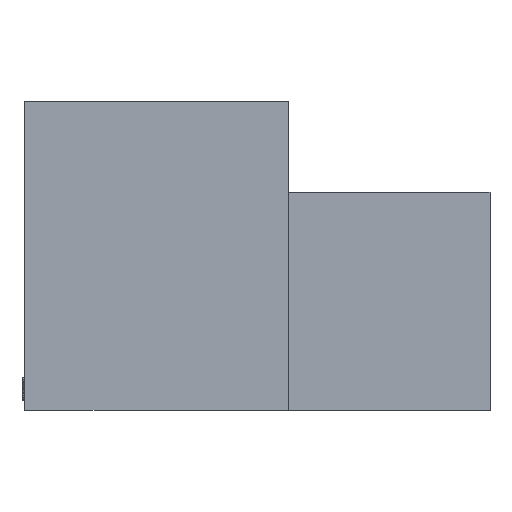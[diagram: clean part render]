
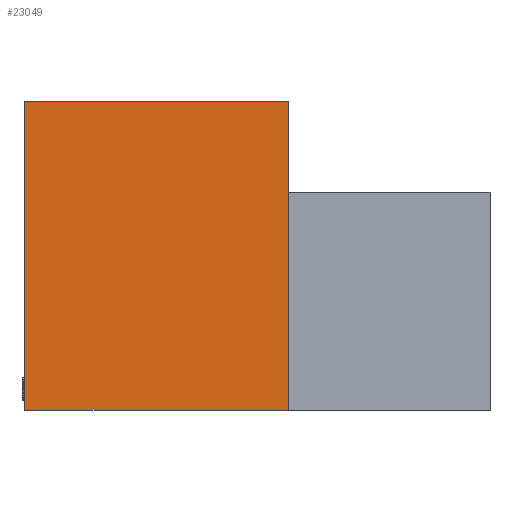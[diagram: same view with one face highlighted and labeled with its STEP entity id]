
A CAD part, left-side view. The second image highlights one B-rep face of the part: STEP entity #23049.
In plain terms, the highlighted planar face has unit normal (-1, 0, 0).
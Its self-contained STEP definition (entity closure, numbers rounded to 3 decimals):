
#2548 = ORIENTED_EDGE ( 'NONE', *, *, #28507, .F. ) ;
#4010 = EDGE_CURVE ( 'NONE', #14065, #12127, #7522, .T. ) ;
#5676 = VECTOR ( 'NONE', #15076, 1000. ) ;
#6004 = CARTESIAN_POINT ( 'NONE',  ( 0., 0., -13.487 ) ) ;
#7060 = CARTESIAN_POINT ( 'NONE',  ( 0., 0., 0. ) ) ;
#7522 = LINE ( 'NONE', #29493, #5676 ) ;
#7609 = CARTESIAN_POINT ( 'NONE',  ( 0., 11.506, 0. ) ) ;
#7716 = LINE ( 'NONE', #26022, #24656 ) ;
#8737 = ORIENTED_EDGE ( 'NONE', *, *, #4010, .F. ) ;
#9044 = EDGE_LOOP ( 'NONE', ( #2548, #8737, #27747, #22302 ) ) ;
#10040 = EDGE_CURVE ( 'NONE', #21466, #14065, #27737, .T. ) ;
#11107 = LINE ( 'NONE', #30777, #28053 ) ;
#12127 = VERTEX_POINT ( 'NONE', #6004 ) ;
#14065 = VERTEX_POINT ( 'NONE', #14375 ) ;
#14375 = CARTESIAN_POINT ( 'NONE',  ( 0., 0., 0. ) ) ;
#15076 = DIRECTION ( 'NONE',  ( 0., 0., -1. ) ) ;
#16360 = DIRECTION ( 'NONE',  ( 0., 1., 0. ) ) ;
#18876 = DIRECTION ( 'NONE',  ( 0., 0., 1. ) ) ;
#19859 = CARTESIAN_POINT ( 'NONE',  ( 0., 11.506, 0. ) ) ;
#21290 = AXIS2_PLACEMENT_3D ( 'NONE', #7060, #28750, #24002 ) ;
#21466 = VERTEX_POINT ( 'NONE', #7609 ) ;
#21581 = PLANE ( 'NONE',  #21290 ) ;
#22302 = ORIENTED_EDGE ( 'NONE', *, *, #28641, .F. ) ;
#22404 = DIRECTION ( 'NONE',  ( 0., -1., 0. ) ) ;
#23049 = ADVANCED_FACE ( 'NONE', ( #23378 ), #21581, .F. ) ;
#23378 = FACE_OUTER_BOUND ( 'NONE', #9044, .T. ) ;
#24002 = DIRECTION ( 'NONE',  ( 0., 0., -1. ) ) ;
#24093 = VERTEX_POINT ( 'NONE', #24475 ) ;
#24475 = CARTESIAN_POINT ( 'NONE',  ( 0., 11.506, -13.487 ) ) ;
#24656 = VECTOR ( 'NONE', #18876, 1000. ) ;
#26022 = CARTESIAN_POINT ( 'NONE',  ( 0., 11.506, -13.487 ) ) ;
#26199 = VECTOR ( 'NONE', #22404, 1000. ) ;
#27737 = LINE ( 'NONE', #19859, #26199 ) ;
#27747 = ORIENTED_EDGE ( 'NONE', *, *, #10040, .F. ) ;
#28053 = VECTOR ( 'NONE', #16360, 1000. ) ;
#28507 = EDGE_CURVE ( 'NONE', #12127, #24093, #11107, .T. ) ;
#28641 = EDGE_CURVE ( 'NONE', #24093, #21466, #7716, .T. ) ;
#28750 = DIRECTION ( 'NONE',  ( 1., 0., 0. ) ) ;
#29493 = CARTESIAN_POINT ( 'NONE',  ( 0., 0., 0. ) ) ;
#30777 = CARTESIAN_POINT ( 'NONE',  ( 0., -8.814, -13.487 ) ) ;
